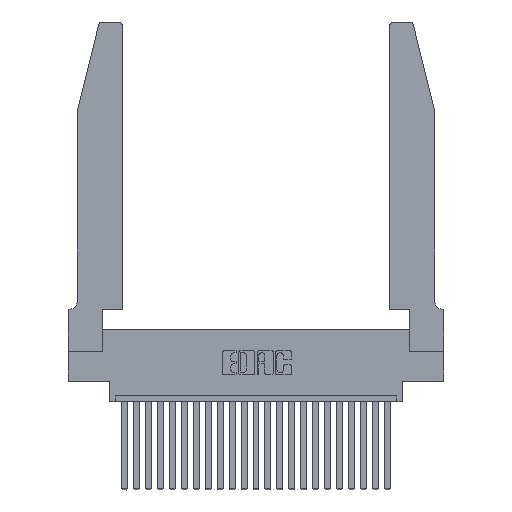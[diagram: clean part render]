
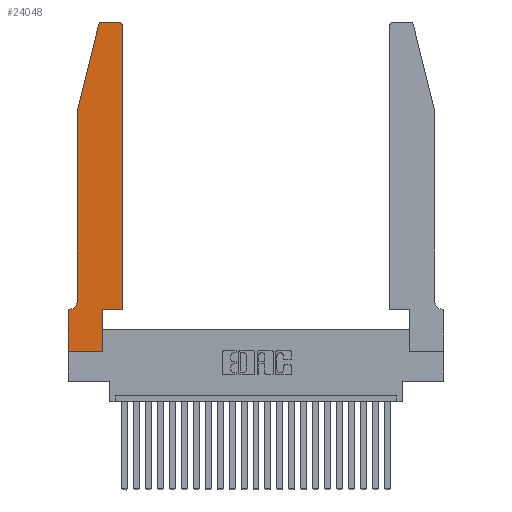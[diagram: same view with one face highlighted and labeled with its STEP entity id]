
A CAD part, top view. The second image highlights one B-rep face of the part: STEP entity #24048.
In plain terms, the highlighted planar face has unit normal (0, 0, 1).
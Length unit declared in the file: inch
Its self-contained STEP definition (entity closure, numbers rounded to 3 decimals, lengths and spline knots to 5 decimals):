
#153 = VECTOR ( 'NONE', #13967, 39.37008 ) ;
#239 = LINE ( 'NONE', #19000, #4103 ) ;
#744 = EDGE_CURVE ( 'NONE', #1083, #21556, #18124, .T. ) ;
#817 = EDGE_CURVE ( 'NONE', #21388, #1161, #19031, .T. ) ;
#933 = LINE ( 'NONE', #12025, #2128 ) ;
#1083 = VERTEX_POINT ( 'NONE', #4802 ) ;
#1144 = EDGE_LOOP ( 'NONE', ( #19442, #15254, #12398, #8693, #5701, #2782, #23591, #21377, #21703, #17481, #2633, #24547 ) ) ;
#1161 = VERTEX_POINT ( 'NONE', #16550 ) ;
#1189 = FACE_OUTER_BOUND ( 'NONE', #1144, .T. ) ;
#1200 = CARTESIAN_POINT ( 'NONE',  ( 0.0755, 0.42, 0.37 ) ) ;
#1242 = CARTESIAN_POINT ( 'NONE',  ( 0.4505, 0.35, 0.37 ) ) ;
#1948 = AXIS2_PLACEMENT_3D ( 'NONE', #5485, #12967, #18914 ) ;
#2128 = VECTOR ( 'NONE', #4364, 39.37008 ) ;
#2209 = DIRECTION ( 'NONE',  ( 0., -1., 0. ) ) ;
#2633 = ORIENTED_EDGE ( 'NONE', *, *, #21106, .T. ) ;
#2780 = CARTESIAN_POINT ( 'NONE',  ( 0.2605, 2.75, 0.37 ) ) ;
#2782 = ORIENTED_EDGE ( 'NONE', *, *, #744, .T. ) ;
#2852 = DIRECTION ( 'NONE',  ( 1., 0., 0. ) ) ;
#2908 = AXIS2_PLACEMENT_3D ( 'NONE', #14157, #6276, #2852 ) ;
#3085 = VERTEX_POINT ( 'NONE', #15061 ) ;
#4103 = VECTOR ( 'NONE', #2209, 39.37008 ) ;
#4364 = DIRECTION ( 'NONE',  ( 1., 0., 0. ) ) ;
#4802 = CARTESIAN_POINT ( 'NONE',  ( 0.0055, 0.35, 0.37 ) ) ;
#4883 = VERTEX_POINT ( 'NONE', #16116 ) ;
#4926 = CIRCLE ( 'NONE', #2908, 0.03 ) ;
#5177 = CARTESIAN_POINT ( 'NONE',  ( 0.2865, 0.35, 0.37 ) ) ;
#5376 = DIRECTION ( 'NONE',  ( 1., 0., 0. ) ) ;
#5485 = CARTESIAN_POINT ( 'NONE',  ( 0., 0.35, 0.37 ) ) ;
#5701 = ORIENTED_EDGE ( 'NONE', *, *, #8778, .T. ) ;
#5885 = LINE ( 'NONE', #2780, #16639 ) ;
#5914 = VERTEX_POINT ( 'NONE', #1200 ) ;
#6276 = DIRECTION ( 'NONE',  ( 0., 0., 1. ) ) ;
#6475 = CARTESIAN_POINT ( 'NONE',  ( 0.0755, 0.35, 0.37 ) ) ;
#6493 = EDGE_CURVE ( 'NONE', #4883, #21388, #23239, .T. ) ;
#6960 = CARTESIAN_POINT ( 'NONE',  ( 0.0055, 0.42, 0.37 ) ) ;
#7444 = AXIS2_PLACEMENT_3D ( 'NONE', #6960, #20298, #23793 ) ;
#8256 = VECTOR ( 'NONE', #5376, 39.37008 ) ;
#8693 = ORIENTED_EDGE ( 'NONE', *, *, #10538, .T. ) ;
#8778 = EDGE_CURVE ( 'NONE', #5914, #1083, #17216, .T. ) ;
#9083 = DIRECTION ( 'NONE',  ( 0., 1., 0. ) ) ;
#9216 = CARTESIAN_POINT ( 'NONE',  ( 0., 0., 0.37 ) ) ;
#9309 = CARTESIAN_POINT ( 'NONE',  ( 0.2865, 0.35, 0.37 ) ) ;
#9440 = CARTESIAN_POINT ( 'NONE',  ( 0.4505, 0.35, 0.37 ) ) ;
#9601 = DIRECTION ( 'NONE',  ( 0., -1., 0. ) ) ;
#9708 = DIRECTION ( 'NONE',  ( 0., 0., 1. ) ) ;
#10538 = EDGE_CURVE ( 'NONE', #16642, #5914, #14293, .T. ) ;
#11829 = CARTESIAN_POINT ( 'NONE',  ( 0.4505, 2.72, 0.37 ) ) ;
#11962 = DIRECTION ( 'NONE',  ( 1., 0., 0. ) ) ;
#12025 = CARTESIAN_POINT ( 'NONE',  ( 0., 0., 0.37 ) ) ;
#12056 = LINE ( 'NONE', #23429, #153 ) ;
#12398 = ORIENTED_EDGE ( 'NONE', *, *, #14379, .T. ) ;
#12492 = EDGE_CURVE ( 'NONE', #21556, #21752, #239, .T. ) ;
#12863 = EDGE_CURVE ( 'NONE', #3085, #22768, #5885, .T. ) ;
#12926 = AXIS2_PLACEMENT_3D ( 'NONE', #13622, #9708, #11962 ) ;
#12967 = DIRECTION ( 'NONE',  ( 0., 0., 1. ) ) ;
#13622 = CARTESIAN_POINT ( 'NONE',  ( 0.4205, 2.72, 0.37 ) ) ;
#13967 = DIRECTION ( 'NONE',  ( -0.239, -0.971, 0. ) ) ;
#14157 = CARTESIAN_POINT ( 'NONE',  ( 0.284, 2.72, 0.37 ) ) ;
#14190 = DIRECTION ( 'NONE',  ( -1., 0., 0. ) ) ;
#14293 = LINE ( 'NONE', #17129, #19992 ) ;
#14379 = EDGE_CURVE ( 'NONE', #22689, #16642, #12056, .T. ) ;
#15039 = PLANE ( 'NONE',  #1948 ) ;
#15061 = CARTESIAN_POINT ( 'NONE',  ( 0.4205, 2.75, 0.37 ) ) ;
#15254 = ORIENTED_EDGE ( 'NONE', *, *, #23247, .T. ) ;
#16116 = CARTESIAN_POINT ( 'NONE',  ( 0.2865, 0., 0.37 ) ) ;
#16550 = CARTESIAN_POINT ( 'NONE',  ( 0.4505, 0.35, 0.37 ) ) ;
#16639 = VECTOR ( 'NONE', #21929, 39.37008 ) ;
#16642 = VERTEX_POINT ( 'NONE', #22140 ) ;
#16658 = CARTESIAN_POINT ( 'NONE',  ( 0.284, 2.75, 0.37 ) ) ;
#17085 = CIRCLE ( 'NONE', #12926, 0.03 ) ;
#17129 = CARTESIAN_POINT ( 'NONE',  ( 0.0755, 2., 0.37 ) ) ;
#17216 = CIRCLE ( 'NONE', #7444, 0.07 ) ;
#17481 = ORIENTED_EDGE ( 'NONE', *, *, #817, .T. ) ;
#17523 = CARTESIAN_POINT ( 'NONE',  ( 0.25487, 2.72718, 0.37 ) ) ;
#18124 = LINE ( 'NONE', #6475, #21348 ) ;
#18605 = VECTOR ( 'NONE', #23690, 39.37008 ) ;
#18914 = DIRECTION ( 'NONE',  ( 1., 0., 0. ) ) ;
#19000 = CARTESIAN_POINT ( 'NONE',  ( 0., 0., 0.37 ) ) ;
#19031 = LINE ( 'NONE', #9440, #8256 ) ;
#19258 = CARTESIAN_POINT ( 'NONE',  ( 0., 0.35, 0.37 ) ) ;
#19442 = ORIENTED_EDGE ( 'NONE', *, *, #12863, .T. ) ;
#19722 = VECTOR ( 'NONE', #9083, 39.37008 ) ;
#19992 = VECTOR ( 'NONE', #9601, 39.37008 ) ;
#20298 = DIRECTION ( 'NONE',  ( 0., 0., -1. ) ) ;
#21106 = EDGE_CURVE ( 'NONE', #1161, #22751, #23595, .T. ) ;
#21348 = VECTOR ( 'NONE', #14190, 39.37008 ) ;
#21377 = ORIENTED_EDGE ( 'NONE', *, *, #22011, .T. ) ;
#21388 = VERTEX_POINT ( 'NONE', #9309 ) ;
#21431 = EDGE_CURVE ( 'NONE', #22751, #3085, #17085, .T. ) ;
#21556 = VERTEX_POINT ( 'NONE', #19258 ) ;
#21703 = ORIENTED_EDGE ( 'NONE', *, *, #6493, .T. ) ;
#21752 = VERTEX_POINT ( 'NONE', #9216 ) ;
#21929 = DIRECTION ( 'NONE',  ( -1., 0., 0. ) ) ;
#22011 = EDGE_CURVE ( 'NONE', #21752, #4883, #933, .T. ) ;
#22140 = CARTESIAN_POINT ( 'NONE',  ( 0.0755, 2., 0.37 ) ) ;
#22689 = VERTEX_POINT ( 'NONE', #17523 ) ;
#22751 = VERTEX_POINT ( 'NONE', #11829 ) ;
#22768 = VERTEX_POINT ( 'NONE', #16658 ) ;
#23239 = LINE ( 'NONE', #5177, #19722 ) ;
#23247 = EDGE_CURVE ( 'NONE', #22768, #22689, #4926, .T. ) ;
#23429 = CARTESIAN_POINT ( 'NONE',  ( 0.0755, 2., 0.37 ) ) ;
#23591 = ORIENTED_EDGE ( 'NONE', *, *, #12492, .T. ) ;
#23595 = LINE ( 'NONE', #1242, #18605 ) ;
#23690 = DIRECTION ( 'NONE',  ( 0., 1., 0. ) ) ;
#23793 = DIRECTION ( 'NONE',  ( -1., 0., 0. ) ) ;
#24048 = ADVANCED_FACE ( 'NONE', ( #1189 ), #15039, .T. ) ;
#24547 = ORIENTED_EDGE ( 'NONE', *, *, #21431, .T. ) ;
